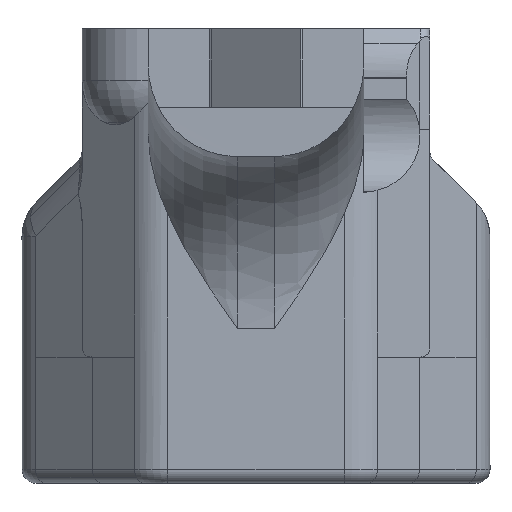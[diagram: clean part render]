
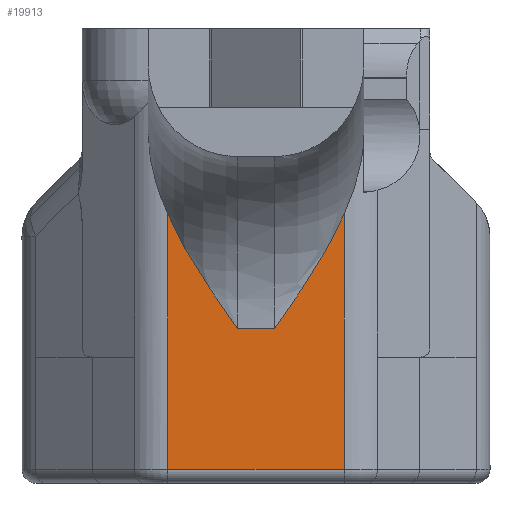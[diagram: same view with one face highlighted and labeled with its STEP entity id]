
A CAD part, front view. The second image highlights one B-rep face of the part: STEP entity #19913.
In plain terms, the highlighted planar face has unit normal (0, -1, 0).
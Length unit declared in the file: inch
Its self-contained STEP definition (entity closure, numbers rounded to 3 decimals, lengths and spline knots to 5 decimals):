
#262 = CARTESIAN_POINT ( 'NONE',  ( 1.03975, 0.585, -3.76359 ) ) ;
#626 = EDGE_CURVE ( 'NONE', #16874, #12648, #16220, .T. ) ;
#852 = VECTOR ( 'NONE', #18303, 39.37008 ) ;
#887 = CARTESIAN_POINT ( 'NONE',  ( 0.51514, 0.585, -3.91784 ) ) ;
#959 = CARTESIAN_POINT ( 'NONE',  ( 0.40534, 0.585, -3.73411 ) ) ;
#1193 = CARTESIAN_POINT ( 'NONE',  ( 1.10256, 0.585, -3.63546 ) ) ;
#1288 = CARTESIAN_POINT ( 'NONE',  ( 0.92748, 0.585, -3.94681 ) ) ;
#1635 = VERTEX_POINT ( 'NONE', #13880 ) ;
#1918 = CARTESIAN_POINT ( 'NONE',  ( 1.03036, 0.585, -3.78049 ) ) ;
#2268 = VERTEX_POINT ( 'NONE', #19750 ) ;
#2315 = ORIENTED_EDGE ( 'NONE', *, *, #10624, .T. ) ;
#2628 = CARTESIAN_POINT ( 'NONE',  ( 0.35938, 0.585, -3.63547 ) ) ;
#2776 = DIRECTION ( 'NONE',  ( 0., 0., 1. ) ) ;
#3089 = VECTOR ( 'NONE', #7124, 39.37008 ) ;
#3574 = CARTESIAN_POINT ( 'NONE',  ( 1.02808, 0.585, -3.78452 ) ) ;
#3921 = VERTEX_POINT ( 'NONE', #8353 ) ;
#4797 = CARTESIAN_POINT ( 'NONE',  ( 0.53445, 0.585, -3.94681 ) ) ;
#4834 = DIRECTION ( 'NONE',  ( 1., 0., 0. ) ) ;
#4870 = LINE ( 'NONE', #13391, #8703 ) ;
#5134 = EDGE_CURVE ( 'NONE', #6711, #1635, #14087, .T. ) ;
#5245 = CARTESIAN_POINT ( 'NONE',  ( 0.9993, 0.585, -3.83539 ) ) ;
#5553 = CARTESIAN_POINT ( 'NONE',  ( 0.35938, 0.585, -4.76846 ) ) ;
#5840 = CARTESIAN_POINT ( 'NONE',  ( 1.10256, 0.585, -4.70941 ) ) ;
#5871 = CARTESIAN_POINT ( 'NONE',  ( 0.48816, 0.585, -3.87598 ) ) ;
#6197 = ORIENTED_EDGE ( 'NONE', *, *, #9931, .T. ) ;
#6711 = VERTEX_POINT ( 'NONE', #9709 ) ;
#6800 = CARTESIAN_POINT ( 'NONE',  ( 1.10256, 0.585, -4.238 ) ) ;
#6883 = CARTESIAN_POINT ( 'NONE',  ( 0.92748, 0.585, -3.94681 ) ) ;
#6997 = EDGE_CURVE ( 'NONE', #11091, #16874, #20059, .T. ) ;
#7124 = DIRECTION ( 'NONE',  ( 0., 0., -1. ) ) ;
#7133 = CARTESIAN_POINT ( 'NONE',  ( 0.35938, 0.585, -3.63547 ) ) ;
#7539 = CARTESIAN_POINT ( 'NONE',  ( 0.44706, 0.585, -3.80759 ) ) ;
#7800 = ORIENTED_EDGE ( 'NONE', *, *, #5134, .F. ) ;
#8114 = CARTESIAN_POINT ( 'NONE',  ( 0.61287, 0.585, -4.06096 ) ) ;
#8120 = FACE_OUTER_BOUND ( 'NONE', #13152, .T. ) ;
#8353 = CARTESIAN_POINT ( 'NONE',  ( 0.80909, 0.585, -4.1175 ) ) ;
#8665 = B_SPLINE_CURVE_WITH_KNOTS ( 'NONE', 3,
 ( #1193, #16021, #19979, #10130, #262, #11773, #1918, #13423, #3574, #15082, #5245, #16723, #6883 ),
 .UNSPECIFIED., .F., .F.,
 ( 4, 1, 1, 1, 1, 1, 2, 2, 4 ),
 ( 0., 0.25, 0.375, 0.4375, 0.46875, 0.48438, 0.49219, 0.5, 1. ),
 .UNSPECIFIED. ) ;
#8703 = VECTOR ( 'NONE', #13517, 39.37008 ) ;
#9120 = CARTESIAN_POINT ( 'NONE',  ( 1.18409, 0.585, 3.265 ) ) ;
#9184 = CARTESIAN_POINT ( 'NONE',  ( 0.43805, 0.585, -3.79192 ) ) ;
#9518 = CARTESIAN_POINT ( 'NONE',  ( 0.84907, 0.585, -4.06096 ) ) ;
#9704 = CARTESIAN_POINT ( 'NONE',  ( 0.57288, 0.585, -4.00442 ) ) ;
#9709 = CARTESIAN_POINT ( 'NONE',  ( 0.53445, 0.585, -3.94681 ) ) ;
#9931 = EDGE_CURVE ( 'NONE', #3921, #1635, #4870, .T. ) ;
#10130 = CARTESIAN_POINT ( 'NONE',  ( 1.05188, 0.585, -3.7412 ) ) ;
#10335 = EDGE_CURVE ( 'NONE', #3921, #19848, #13662, .T. ) ;
#10624 = EDGE_CURVE ( 'NONE', #6711, #11091, #12072, .T. ) ;
#10832 = CARTESIAN_POINT ( 'NONE',  ( 0.43544, 0.585, -3.78733 ) ) ;
#10978 = PLANE ( 'NONE',  #16455 ) ;
#11091 = VERTEX_POINT ( 'NONE', #7133 ) ;
#11148 = CARTESIAN_POINT ( 'NONE',  ( 0.88906, 0.585, -4.00442 ) ) ;
#11334 = ORIENTED_EDGE ( 'NONE', *, *, #6997, .T. ) ;
#11773 = CARTESIAN_POINT ( 'NONE',  ( 1.03352, 0.585, -3.77484 ) ) ;
#12040 = ORIENTED_EDGE ( 'NONE', *, *, #19474, .T. ) ;
#12072 = B_SPLINE_CURVE_WITH_KNOTS ( 'NONE', 3,
 ( #20611, #887, #5871, #17362, #7539, #19029, #9184, #20688, #10832, #959, #12472, #2628 ),
 .UNSPECIFIED., .F., .F.,
 ( 4, 1, 1, 1, 1, 2, 2, 4 ),
 ( 0., 0.25, 0.375, 0.4375, 0.46875, 0.48437, 0.5, 1. ),
 .UNSPECIFIED. ) ;
#12472 = CARTESIAN_POINT ( 'NONE',  ( 0.38029, 0.585, -3.68403 ) ) ;
#12631 = DIRECTION ( 'NONE',  ( 0., -1., 0. ) ) ;
#12648 = VERTEX_POINT ( 'NONE', #5840 ) ;
#13141 = EDGE_CURVE ( 'NONE', #2268, #19848, #8665, .T. ) ;
#13152 = EDGE_LOOP ( 'NONE', ( #11334, #17463, #12040, #14173, #19860, #6197, #7800, #2315 ) ) ;
#13391 = CARTESIAN_POINT ( 'NONE',  ( 1.18409, 0.585, -4.1175 ) ) ;
#13423 = CARTESIAN_POINT ( 'NONE',  ( 1.029, 0.585, -3.78291 ) ) ;
#13491 = LINE ( 'NONE', #6800, #852 ) ;
#13517 = DIRECTION ( 'NONE',  ( -1., 0., 0. ) ) ;
#13662 = B_SPLINE_CURVE_WITH_KNOTS ( 'NONE', 3,
 ( #19280, #9518, #11148, #1288 ),
 .UNSPECIFIED., .F., .F.,
 ( 4, 4 ),
 ( -0.00003, 0.00525 ),
 .UNSPECIFIED. ) ;
#13880 = CARTESIAN_POINT ( 'NONE',  ( 0.65284, 0.585, -4.1175 ) ) ;
#14087 = B_SPLINE_CURVE_WITH_KNOTS ( 'NONE', 3,
 ( #4797, #9704, #8114, #19619 ),
 .UNSPECIFIED., .F., .F.,
 ( 4, 4 ),
 ( 0.00052, 0.0058 ),
 .UNSPECIFIED. ) ;
#14173 = ORIENTED_EDGE ( 'NONE', *, *, #13141, .T. ) ;
#15082 = CARTESIAN_POINT ( 'NONE',  ( 1.02761, 0.585, -3.78537 ) ) ;
#15149 = CARTESIAN_POINT ( 'NONE',  ( 0.35938, 0.585, -4.70941 ) ) ;
#16021 = CARTESIAN_POINT ( 'NONE',  ( 1.09207, 0.585, -3.65981 ) ) ;
#16220 = LINE ( 'NONE', #17486, #20571 ) ;
#16455 = AXIS2_PLACEMENT_3D ( 'NONE', #9120, #12631, #2776 ) ;
#16723 = CARTESIAN_POINT ( 'NONE',  ( 0.96608, 0.585, -3.88894 ) ) ;
#16874 = VERTEX_POINT ( 'NONE', #15149 ) ;
#17362 = CARTESIAN_POINT ( 'NONE',  ( 0.46018, 0.585, -3.82992 ) ) ;
#17463 = ORIENTED_EDGE ( 'NONE', *, *, #626, .T. ) ;
#17486 = CARTESIAN_POINT ( 'NONE',  ( 1.18409, 0.585, -4.70941 ) ) ;
#18303 = DIRECTION ( 'NONE',  ( 0., 0., 1. ) ) ;
#19029 = CARTESIAN_POINT ( 'NONE',  ( 0.44072, 0.585, -3.79659 ) ) ;
#19280 = CARTESIAN_POINT ( 'NONE',  ( 0.80909, 0.585, -4.1175 ) ) ;
#19474 = EDGE_CURVE ( 'NONE', #12648, #2268, #13491, .T. ) ;
#19619 = CARTESIAN_POINT ( 'NONE',  ( 0.65284, 0.585, -4.1175 ) ) ;
#19750 = CARTESIAN_POINT ( 'NONE',  ( 1.10256, 0.585, -3.63546 ) ) ;
#19848 = VERTEX_POINT ( 'NONE', #20621 ) ;
#19860 = ORIENTED_EDGE ( 'NONE', *, *, #10335, .F. ) ;
#19913 = ADVANCED_FACE ( 'NONE', ( #8120 ), #10978, .T. ) ;
#19979 = CARTESIAN_POINT ( 'NONE',  ( 1.07478, 0.585, -3.69692 ) ) ;
#20059 = LINE ( 'NONE', #5553, #3089 ) ;
#20571 = VECTOR ( 'NONE', #4834, 39.37008 ) ;
#20611 = CARTESIAN_POINT ( 'NONE',  ( 0.53445, 0.585, -3.94681 ) ) ;
#20621 = CARTESIAN_POINT ( 'NONE',  ( 0.92748, 0.585, -3.94681 ) ) ;
#20688 = CARTESIAN_POINT ( 'NONE',  ( 0.43628, 0.585, -3.78881 ) ) ;
